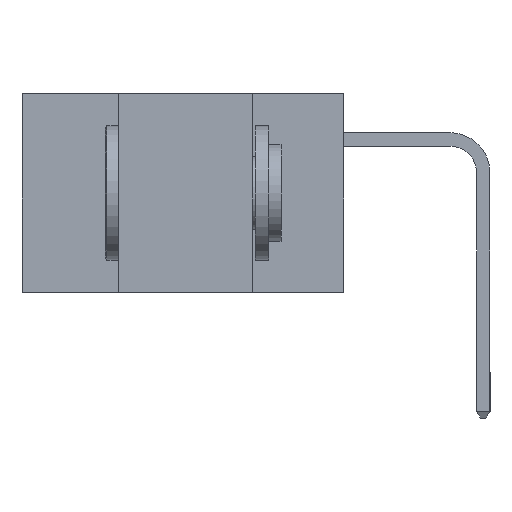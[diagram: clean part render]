
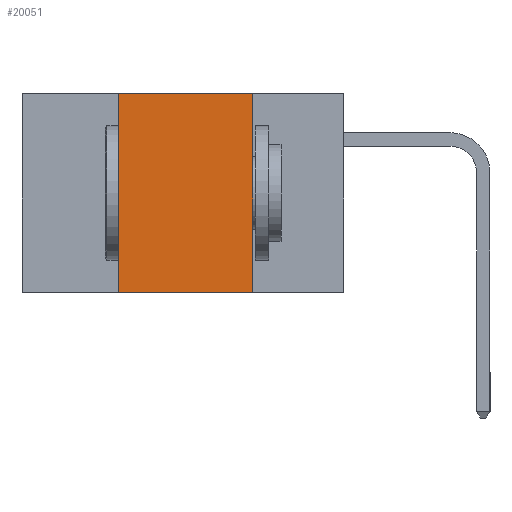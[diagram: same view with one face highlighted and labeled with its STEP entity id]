
A CAD part, left-side view. The second image highlights one B-rep face of the part: STEP entity #20051.
In plain terms, the highlighted planar face has unit normal (-1, 0, 0).
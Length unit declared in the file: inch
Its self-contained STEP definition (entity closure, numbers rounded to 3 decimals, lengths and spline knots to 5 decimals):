
#164 = LINE ( 'NONE', #14306, #15557 ) ;
#1309 = DIRECTION ( 'NONE',  ( 0., 0., -1. ) ) ;
#1710 = CARTESIAN_POINT ( 'NONE',  ( 0., 0.42, -0.37 ) ) ;
#3384 = DIRECTION ( 'NONE',  ( 1., 0., 0. ) ) ;
#3399 = LINE ( 'NONE', #21290, #18902 ) ;
#3868 = VECTOR ( 'NONE', #13664, 39.37008 ) ;
#4556 = ORIENTED_EDGE ( 'NONE', *, *, #7662, .F. ) ;
#4805 = DIRECTION ( 'NONE',  ( 0., 0., -1. ) ) ;
#5060 = CARTESIAN_POINT ( 'NONE',  ( 0., 0.6, 0. ) ) ;
#7314 = ORIENTED_EDGE ( 'NONE', *, *, #23488, .T. ) ;
#7662 = EDGE_CURVE ( 'NONE', #14769, #9523, #18407, .T. ) ;
#8957 = CARTESIAN_POINT ( 'NONE',  ( 0., 0.6, 0. ) ) ;
#9523 = VERTEX_POINT ( 'NONE', #18645 ) ;
#9646 = LINE ( 'NONE', #13551, #3868 ) ;
#11211 = ORIENTED_EDGE ( 'NONE', *, *, #20613, .F. ) ;
#11363 = VERTEX_POINT ( 'NONE', #1710 ) ;
#13551 = CARTESIAN_POINT ( 'NONE',  ( 0., 0.42, -0.37 ) ) ;
#13589 = ORIENTED_EDGE ( 'NONE', *, *, #23853, .F. ) ;
#13664 = DIRECTION ( 'NONE',  ( 0., 0., 1. ) ) ;
#14306 = CARTESIAN_POINT ( 'NONE',  ( 0., 0.6, -0.37 ) ) ;
#14664 = DIRECTION ( 'NONE',  ( 0., -1., 0. ) ) ;
#14671 = FACE_OUTER_BOUND ( 'NONE', #20843, .T. ) ;
#14769 = VERTEX_POINT ( 'NONE', #22134 ) ;
#15557 = VECTOR ( 'NONE', #22204, 39.37008 ) ;
#18407 = LINE ( 'NONE', #8957, #18710 ) ;
#18645 = CARTESIAN_POINT ( 'NONE',  ( 0., 0.17, 0. ) ) ;
#18710 = VECTOR ( 'NONE', #14664, 39.37008 ) ;
#18902 = VECTOR ( 'NONE', #1309, 39.37008 ) ;
#18945 = VERTEX_POINT ( 'NONE', #21314 ) ;
#20051 = ADVANCED_FACE ( 'NONE', ( #14671 ), #21017, .F. ) ;
#20613 = EDGE_CURVE ( 'NONE', #11363, #14769, #9646, .T. ) ;
#20843 = EDGE_LOOP ( 'NONE', ( #13589, #4556, #11211, #7314 ) ) ;
#21017 = PLANE ( 'NONE',  #22887 ) ;
#21290 = CARTESIAN_POINT ( 'NONE',  ( 0., 0.17, -0.37 ) ) ;
#21314 = CARTESIAN_POINT ( 'NONE',  ( 0., 0.17, -0.37 ) ) ;
#22134 = CARTESIAN_POINT ( 'NONE',  ( 0., 0.42, 0. ) ) ;
#22204 = DIRECTION ( 'NONE',  ( 0., -1., 0. ) ) ;
#22887 = AXIS2_PLACEMENT_3D ( 'NONE', #5060, #3384, #4805 ) ;
#23488 = EDGE_CURVE ( 'NONE', #11363, #18945, #164, .T. ) ;
#23853 = EDGE_CURVE ( 'NONE', #9523, #18945, #3399, .T. ) ;
